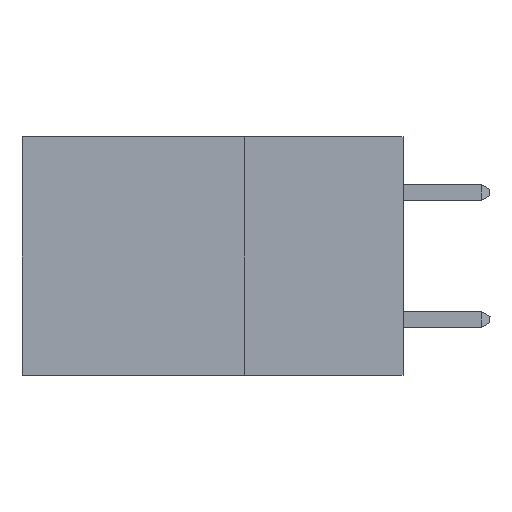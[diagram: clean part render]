
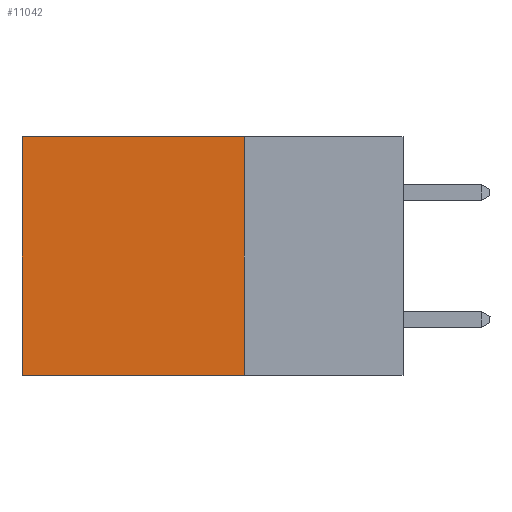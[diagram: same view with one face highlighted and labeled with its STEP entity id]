
A CAD part, left-side view. The second image highlights one B-rep face of the part: STEP entity #11042.
In plain terms, the highlighted planar face has unit normal (-1, 0, 0).
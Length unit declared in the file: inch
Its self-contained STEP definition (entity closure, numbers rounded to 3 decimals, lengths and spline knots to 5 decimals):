
#1028 = VERTEX_POINT ( 'NONE', #5963 ) ;
#1323 = CARTESIAN_POINT ( 'NONE',  ( 0.2875, 0.6, -0.375 ) ) ;
#2073 = EDGE_CURVE ( 'NONE', #6005, #1028, #13169, .T. ) ;
#2349 = DIRECTION ( 'NONE',  ( 0., 0., -1. ) ) ;
#2803 = DIRECTION ( 'NONE',  ( 0., 0., -1. ) ) ;
#3594 = LINE ( 'NONE', #1323, #19540 ) ;
#3947 = CARTESIAN_POINT ( 'NONE',  ( 0.2875, 0.25, 0. ) ) ;
#4254 = DIRECTION ( 'NONE',  ( 0., 1., 0. ) ) ;
#4434 = EDGE_CURVE ( 'NONE', #6005, #13664, #19325, .T. ) ;
#4448 = VECTOR ( 'NONE', #4254, 39.37008 ) ;
#5963 = CARTESIAN_POINT ( 'NONE',  ( 0.2875, 0.6, 0. ) ) ;
#6005 = VERTEX_POINT ( 'NONE', #3947 ) ;
#6080 = ORIENTED_EDGE ( 'NONE', *, *, #11868, .F. ) ;
#6960 = PLANE ( 'NONE',  #9074 ) ;
#8507 = DIRECTION ( 'NONE',  ( 1., 0., 0. ) ) ;
#9074 = AXIS2_PLACEMENT_3D ( 'NONE', #17751, #8507, #2349 ) ;
#9135 = ORIENTED_EDGE ( 'NONE', *, *, #4434, .F. ) ;
#10232 = CARTESIAN_POINT ( 'NONE',  ( 0.2875, 0.25, 0. ) ) ;
#10643 = VECTOR ( 'NONE', #19541, 39.37008 ) ;
#11042 = ADVANCED_FACE ( 'NONE', ( #19539 ), #6960, .F. ) ;
#11731 = DIRECTION ( 'NONE',  ( 0., 1., 0. ) ) ;
#11868 = EDGE_CURVE ( 'NONE', #13664, #14024, #19283, .T. ) ;
#13169 = LINE ( 'NONE', #10232, #4448 ) ;
#13664 = VERTEX_POINT ( 'NONE', #14784 ) ;
#14024 = VERTEX_POINT ( 'NONE', #17131 ) ;
#14784 = CARTESIAN_POINT ( 'NONE',  ( 0.2875, 0.25, -0.375 ) ) ;
#15156 = VECTOR ( 'NONE', #11731, 39.37008 ) ;
#16340 = CARTESIAN_POINT ( 'NONE',  ( 0.2875, 0.25, -0.375 ) ) ;
#17037 = EDGE_CURVE ( 'NONE', #1028, #14024, #3594, .T. ) ;
#17131 = CARTESIAN_POINT ( 'NONE',  ( 0.2875, 0.6, -0.375 ) ) ;
#17751 = CARTESIAN_POINT ( 'NONE',  ( 0.2875, 0.25, -0.375 ) ) ;
#17758 = ORIENTED_EDGE ( 'NONE', *, *, #17037, .T. ) ;
#18282 = EDGE_LOOP ( 'NONE', ( #17758, #6080, #9135, #19339 ) ) ;
#19283 = LINE ( 'NONE', #16340, #15156 ) ;
#19325 = LINE ( 'NONE', #19474, #10643 ) ;
#19339 = ORIENTED_EDGE ( 'NONE', *, *, #2073, .T. ) ;
#19474 = CARTESIAN_POINT ( 'NONE',  ( 0.2875, 0.25, -0.375 ) ) ;
#19539 = FACE_OUTER_BOUND ( 'NONE', #18282, .T. ) ;
#19540 = VECTOR ( 'NONE', #2803, 39.37008 ) ;
#19541 = DIRECTION ( 'NONE',  ( 0., 0., -1. ) ) ;
